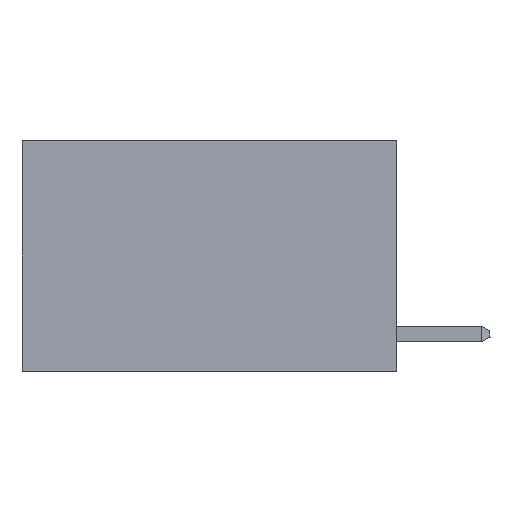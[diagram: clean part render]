
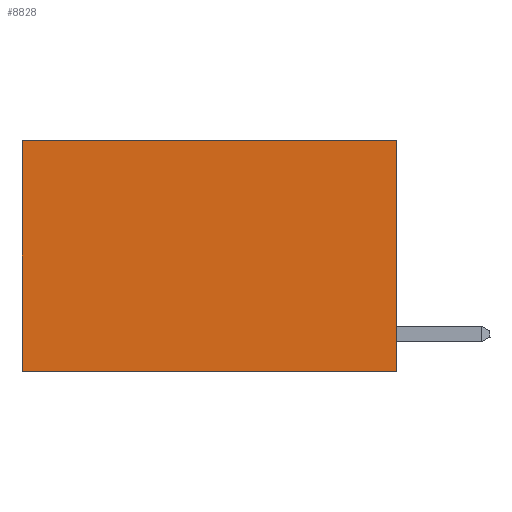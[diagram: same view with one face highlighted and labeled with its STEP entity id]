
A CAD part, left-side view. The second image highlights one B-rep face of the part: STEP entity #8828.
In plain terms, the highlighted planar face has unit normal (-1, 0, 0).
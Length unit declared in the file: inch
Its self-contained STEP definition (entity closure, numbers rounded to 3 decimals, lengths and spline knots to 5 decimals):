
#111 = ORIENTED_EDGE ( 'NONE', *, *, #17937, .F. ) ;
#1549 = ORIENTED_EDGE ( 'NONE', *, *, #14737, .F. ) ;
#2168 = LINE ( 'NONE', #13805, #17525 ) ;
#4368 = CARTESIAN_POINT ( 'NONE',  ( 0.2625, 0., 0. ) ) ;
#4444 = VERTEX_POINT ( 'NONE', #9281 ) ;
#4463 = DIRECTION ( 'NONE',  ( 0., 0., -1. ) ) ;
#4883 = CARTESIAN_POINT ( 'NONE',  ( 0.2625, 0.6, 0. ) ) ;
#5174 = ORIENTED_EDGE ( 'NONE', *, *, #11335, .T. ) ;
#6236 = CARTESIAN_POINT ( 'NONE',  ( 0.2625, 0.6, -0.37 ) ) ;
#7004 = CARTESIAN_POINT ( 'NONE',  ( 0.2625, 0.6, 0. ) ) ;
#8828 = ADVANCED_FACE ( 'NONE', ( #23999 ), #14433, .F. ) ;
#9281 = CARTESIAN_POINT ( 'NONE',  ( 0.2625, 0., 0. ) ) ;
#9875 = DIRECTION ( 'NONE',  ( 0., 0., -1. ) ) ;
#10061 = VERTEX_POINT ( 'NONE', #6236 ) ;
#10258 = LINE ( 'NONE', #7004, #20816 ) ;
#10875 = AXIS2_PLACEMENT_3D ( 'NONE', #4368, #16425, #4463 ) ;
#10931 = DIRECTION ( 'NONE',  ( 0., 1., 0. ) ) ;
#11335 = EDGE_CURVE ( 'NONE', #14151, #10061, #10258, .T. ) ;
#12115 = VECTOR ( 'NONE', #10931, 39.37008 ) ;
#12756 = LINE ( 'NONE', #14773, #12115 ) ;
#13805 = CARTESIAN_POINT ( 'NONE',  ( 0.2625, 0., 0. ) ) ;
#14151 = VERTEX_POINT ( 'NONE', #4883 ) ;
#14433 = PLANE ( 'NONE',  #10875 ) ;
#14737 = EDGE_CURVE ( 'NONE', #18541, #10061, #21693, .T. ) ;
#14773 = CARTESIAN_POINT ( 'NONE',  ( 0.2625, 0., 0. ) ) ;
#16425 = DIRECTION ( 'NONE',  ( 1., 0., 0. ) ) ;
#17525 = VECTOR ( 'NONE', #9875, 39.37008 ) ;
#17937 = EDGE_CURVE ( 'NONE', #4444, #18541, #2168, .T. ) ;
#18541 = VERTEX_POINT ( 'NONE', #21551 ) ;
#20816 = VECTOR ( 'NONE', #20892, 39.37008 ) ;
#20892 = DIRECTION ( 'NONE',  ( 0., 0., -1. ) ) ;
#21075 = VECTOR ( 'NONE', #24751, 39.37008 ) ;
#21551 = CARTESIAN_POINT ( 'NONE',  ( 0.2625, 0., -0.37 ) ) ;
#21693 = LINE ( 'NONE', #22749, #21075 ) ;
#22252 = EDGE_CURVE ( 'NONE', #4444, #14151, #12756, .T. ) ;
#22749 = CARTESIAN_POINT ( 'NONE',  ( 0.2625, 0., -0.37 ) ) ;
#23999 = FACE_OUTER_BOUND ( 'NONE', #24124, .T. ) ;
#24124 = EDGE_LOOP ( 'NONE', ( #5174, #1549, #111, #24178 ) ) ;
#24178 = ORIENTED_EDGE ( 'NONE', *, *, #22252, .T. ) ;
#24751 = DIRECTION ( 'NONE',  ( 0., 1., 0. ) ) ;
